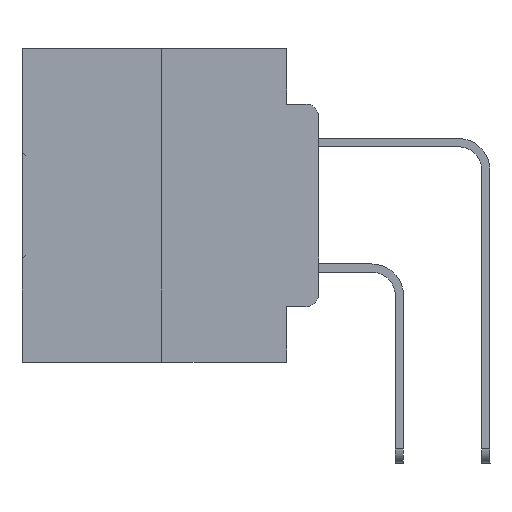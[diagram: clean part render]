
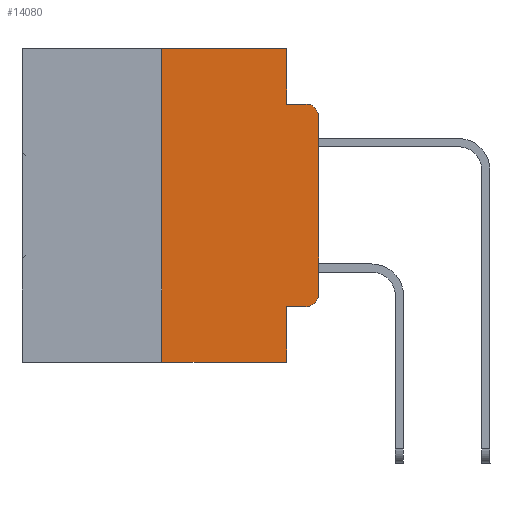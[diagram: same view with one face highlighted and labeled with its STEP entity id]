
A CAD part, left-side view. The second image highlights one B-rep face of the part: STEP entity #14080.
In plain terms, the highlighted planar face has unit normal (-1, 0, 0).
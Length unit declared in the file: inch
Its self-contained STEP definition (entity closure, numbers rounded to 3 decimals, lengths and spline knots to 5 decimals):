
#514 = LINE ( 'NONE', #13008, #18895 ) ;
#1618 = FACE_OUTER_BOUND ( 'NONE', #15762, .T. ) ;
#3040 = LINE ( 'NONE', #9561, #19837 ) ;
#3286 = DIRECTION ( 'NONE',  ( -1., 0., 0. ) ) ;
#4152 = ORIENTED_EDGE ( 'NONE', *, *, #10167, .T. ) ;
#5151 = EDGE_CURVE ( 'NONE', #11019, #19596, #3040, .T. ) ;
#5389 = DIRECTION ( 'NONE',  ( 0., 0., 1. ) ) ;
#5523 = AXIS2_PLACEMENT_3D ( 'NONE', #11872, #29306, #14398 ) ;
#6420 = DIRECTION ( 'NONE',  ( -1., 0., 0. ) ) ;
#6801 = EDGE_CURVE ( 'NONE', #19596, #28913, #20962, .T. ) ;
#8056 = DIRECTION ( 'NONE',  ( 0., -1., 0. ) ) ;
#8463 = EDGE_CURVE ( 'NONE', #11614, #28913, #29792, .T. ) ;
#8539 = VECTOR ( 'NONE', #26795, 39.37008 ) ;
#8820 = CARTESIAN_POINT ( 'NONE',  ( 0., 0.25, -0.5 ) ) ;
#8995 = CARTESIAN_POINT ( 'NONE',  ( 0., 0.051, -0.0885 ) ) ;
#8999 = CARTESIAN_POINT ( 'NONE',  ( 0., 0.02, -0.0885 ) ) ;
#9329 = EDGE_CURVE ( 'NONE', #9664, #11019, #16540, .T. ) ;
#9561 = CARTESIAN_POINT ( 'NONE',  ( 0., 0.051, 0. ) ) ;
#9664 = VERTEX_POINT ( 'NONE', #28532 ) ;
#10167 = EDGE_CURVE ( 'NONE', #12963, #11614, #18794, .T. ) ;
#11019 = VERTEX_POINT ( 'NONE', #23539 ) ;
#11374 = ORIENTED_EDGE ( 'NONE', *, *, #25819, .T. ) ;
#11536 = CARTESIAN_POINT ( 'NONE',  ( 0., 0.473, -0.5 ) ) ;
#11614 = VERTEX_POINT ( 'NONE', #24994 ) ;
#11872 = CARTESIAN_POINT ( 'NONE',  ( 0., 0.473, 0. ) ) ;
#12326 = ORIENTED_EDGE ( 'NONE', *, *, #5151, .F. ) ;
#12782 = VECTOR ( 'NONE', #30037, 39.37008 ) ;
#12963 = VERTEX_POINT ( 'NONE', #25773 ) ;
#13008 = CARTESIAN_POINT ( 'NONE',  ( 0., 0.051, -0.4115 ) ) ;
#13893 = VERTEX_POINT ( 'NONE', #24076 ) ;
#14061 = DIRECTION ( 'NONE',  ( 0., -1., 0. ) ) ;
#14080 = ADVANCED_FACE ( 'NONE', ( #1618 ), #26807, .F. ) ;
#14165 = LINE ( 'NONE', #11536, #20007 ) ;
#14398 = DIRECTION ( 'NONE',  ( 0., 0., -1. ) ) ;
#14713 = CARTESIAN_POINT ( 'NONE',  ( 0., 0.473, 0. ) ) ;
#15292 = VECTOR ( 'NONE', #20040, 39.37008 ) ;
#15395 = CARTESIAN_POINT ( 'NONE',  ( 0., 0.051, -0.4115 ) ) ;
#15762 = EDGE_LOOP ( 'NONE', ( #4152, #16368, #22013, #12326, #32213, #21881, #23475, #27481, #23825, #11374 ) ) ;
#16077 = LINE ( 'NONE', #17563, #15292 ) ;
#16368 = ORIENTED_EDGE ( 'NONE', *, *, #8463, .T. ) ;
#16382 = VERTEX_POINT ( 'NONE', #28646 ) ;
#16540 = LINE ( 'NONE', #14713, #28954 ) ;
#16816 = CARTESIAN_POINT ( 'NONE',  ( 0., 0.25, 0. ) ) ;
#17258 = DIRECTION ( 'NONE',  ( 0., -1., 0. ) ) ;
#17473 = VERTEX_POINT ( 'NONE', #15395 ) ;
#17563 = CARTESIAN_POINT ( 'NONE',  ( 0., 0.051, 0. ) ) ;
#18287 = CARTESIAN_POINT ( 'NONE',  ( 0., 0.02, -0.1085 ) ) ;
#18794 = LINE ( 'NONE', #20452, #31176 ) ;
#18895 = VECTOR ( 'NONE', #8056, 39.37008 ) ;
#18896 = VERTEX_POINT ( 'NONE', #8820 ) ;
#19594 = EDGE_CURVE ( 'NONE', #18896, #16382, #14165, .T. ) ;
#19596 = VERTEX_POINT ( 'NONE', #8995 ) ;
#19837 = VECTOR ( 'NONE', #23716, 39.37008 ) ;
#20007 = VECTOR ( 'NONE', #14061, 39.37008 ) ;
#20040 = DIRECTION ( 'NONE',  ( 0., 0., -1. ) ) ;
#20164 = CARTESIAN_POINT ( 'NONE',  ( 0., 0.051, -0.0885 ) ) ;
#20452 = CARTESIAN_POINT ( 'NONE',  ( 0., 0., 0. ) ) ;
#20751 = DIRECTION ( 'NONE',  ( 0., 0., -1. ) ) ;
#20962 = LINE ( 'NONE', #20164, #12782 ) ;
#21366 = CARTESIAN_POINT ( 'NONE',  ( 0., 0.02, -0.3915 ) ) ;
#21881 = ORIENTED_EDGE ( 'NONE', *, *, #30775, .F. ) ;
#22013 = ORIENTED_EDGE ( 'NONE', *, *, #6801, .F. ) ;
#23287 = CIRCLE ( 'NONE', #26900, 0.02 ) ;
#23475 = ORIENTED_EDGE ( 'NONE', *, *, #19594, .T. ) ;
#23539 = CARTESIAN_POINT ( 'NONE',  ( 0., 0.051, 0. ) ) ;
#23716 = DIRECTION ( 'NONE',  ( 0., 0., -1. ) ) ;
#23825 = ORIENTED_EDGE ( 'NONE', *, *, #27523, .T. ) ;
#23874 = DIRECTION ( 'NONE',  ( 0., 0., -1. ) ) ;
#24076 = CARTESIAN_POINT ( 'NONE',  ( 0., 0.02, -0.4115 ) ) ;
#24994 = CARTESIAN_POINT ( 'NONE',  ( 0., 0., -0.1085 ) ) ;
#25773 = CARTESIAN_POINT ( 'NONE',  ( 0., 0., -0.3915 ) ) ;
#25819 = EDGE_CURVE ( 'NONE', #13893, #12963, #23287, .T. ) ;
#26795 = DIRECTION ( 'NONE',  ( 0., 0., 1. ) ) ;
#26807 = PLANE ( 'NONE',  #5523 ) ;
#26900 = AXIS2_PLACEMENT_3D ( 'NONE', #21366, #6420, #23874 ) ;
#27392 = AXIS2_PLACEMENT_3D ( 'NONE', #18287, #3286, #20751 ) ;
#27481 = ORIENTED_EDGE ( 'NONE', *, *, #29150, .F. ) ;
#27523 = EDGE_CURVE ( 'NONE', #17473, #13893, #514, .T. ) ;
#28470 = LINE ( 'NONE', #16816, #8539 ) ;
#28532 = CARTESIAN_POINT ( 'NONE',  ( 0., 0.25, 0. ) ) ;
#28646 = CARTESIAN_POINT ( 'NONE',  ( 0., 0.051, -0.5 ) ) ;
#28913 = VERTEX_POINT ( 'NONE', #8999 ) ;
#28954 = VECTOR ( 'NONE', #17258, 39.37008 ) ;
#29150 = EDGE_CURVE ( 'NONE', #17473, #16382, #16077, .T. ) ;
#29306 = DIRECTION ( 'NONE',  ( 1., 0., 0. ) ) ;
#29792 = CIRCLE ( 'NONE', #27392, 0.02 ) ;
#30037 = DIRECTION ( 'NONE',  ( 0., -1., 0. ) ) ;
#30775 = EDGE_CURVE ( 'NONE', #18896, #9664, #28470, .T. ) ;
#31176 = VECTOR ( 'NONE', #5389, 39.37008 ) ;
#32213 = ORIENTED_EDGE ( 'NONE', *, *, #9329, .F. ) ;
